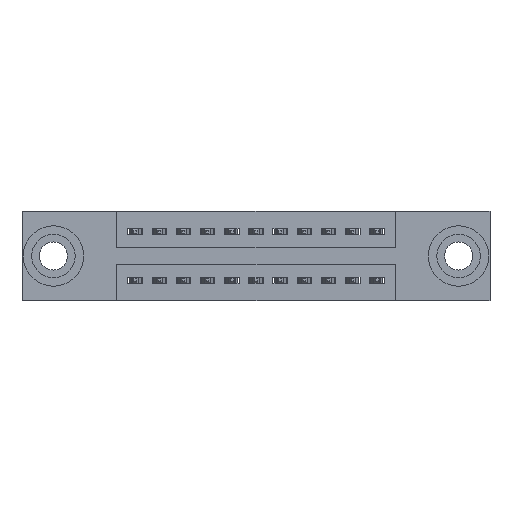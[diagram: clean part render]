
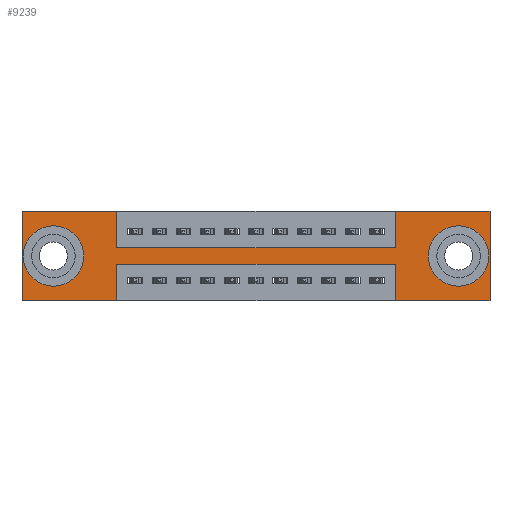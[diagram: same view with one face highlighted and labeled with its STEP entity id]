
A CAD part, front view. The second image highlights one B-rep face of the part: STEP entity #9239.
In plain terms, the highlighted planar face has unit normal (0, -1, 0).
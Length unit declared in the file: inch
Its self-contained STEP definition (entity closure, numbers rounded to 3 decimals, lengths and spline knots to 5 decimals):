
#27 = ORIENTED_EDGE ( 'NONE', *, *, #8693, .F. ) ;
#55 = LINE ( 'NONE', #4113, #10919 ) ;
#176 = CARTESIAN_POINT ( 'NONE',  ( 1.805, 0., -0.263 ) ) ;
#254 = DIRECTION ( 'NONE',  ( 0., 1., 0. ) ) ;
#573 = EDGE_CURVE ( 'NONE', #13334, #4779, #3829, .T. ) ;
#796 = VERTEX_POINT ( 'NONE', #4320 ) ;
#838 = VECTOR ( 'NONE', #10390, 39.37008 ) ;
#892 = CARTESIAN_POINT ( 'NONE',  ( 0.3925, 0., -0.22 ) ) ;
#930 = CARTESIAN_POINT ( 'NONE',  ( 0., 0., 0. ) ) ;
#1156 = CARTESIAN_POINT ( 'NONE',  ( 0., 0., -0.37 ) ) ;
#1163 = EDGE_LOOP ( 'NONE', ( #5607, #6394 ) ) ;
#1349 = VERTEX_POINT ( 'NONE', #5941 ) ;
#1378 = DIRECTION ( 'NONE',  ( 0., 0., 1. ) ) ;
#1392 = EDGE_CURVE ( 'NONE', #10731, #13496, #9071, .T. ) ;
#1837 = CARTESIAN_POINT ( 'NONE',  ( 0.3925, 0., -0.15 ) ) ;
#1851 = DIRECTION ( 'NONE',  ( 1., 0., 0. ) ) ;
#1896 = EDGE_CURVE ( 'NONE', #3191, #8686, #5848, .T. ) ;
#1983 = ORIENTED_EDGE ( 'NONE', *, *, #9876, .F. ) ;
#2109 = CARTESIAN_POINT ( 'NONE',  ( 0.3925, 0., -0.15 ) ) ;
#2482 = EDGE_CURVE ( 'NONE', #2484, #11523, #7688, .T. ) ;
#2484 = VERTEX_POINT ( 'NONE', #2109 ) ;
#2642 = CIRCLE ( 'NONE', #4278, 0.078 ) ;
#2674 = ORIENTED_EDGE ( 'NONE', *, *, #5339, .F. ) ;
#2842 = ORIENTED_EDGE ( 'NONE', *, *, #573, .F. ) ;
#2882 = EDGE_CURVE ( 'NONE', #11814, #8752, #55, .T. ) ;
#3098 = VERTEX_POINT ( 'NONE', #6327 ) ;
#3191 = VERTEX_POINT ( 'NONE', #176 ) ;
#3292 = VECTOR ( 'NONE', #3511, 39.37008 ) ;
#3360 = EDGE_CURVE ( 'NONE', #13496, #4398, #11506, .T. ) ;
#3401 = DIRECTION ( 'NONE',  ( 0., 0., -1. ) ) ;
#3511 = DIRECTION ( 'NONE',  ( 1., 0., 0. ) ) ;
#3582 = FACE_OUTER_BOUND ( 'NONE', #8146, .T. ) ;
#3628 = CARTESIAN_POINT ( 'NONE',  ( 0.3925, 0., 0. ) ) ;
#3829 = LINE ( 'NONE', #10468, #838 ) ;
#4071 = EDGE_CURVE ( 'NONE', #11523, #10731, #13058, .T. ) ;
#4113 = CARTESIAN_POINT ( 'NONE',  ( 0., 0., -0.37 ) ) ;
#4177 = CARTESIAN_POINT ( 'NONE',  ( 1.5425, 0., -0.15 ) ) ;
#4278 = AXIS2_PLACEMENT_3D ( 'NONE', #9083, #9059, #9030 ) ;
#4320 = CARTESIAN_POINT ( 'NONE',  ( 0.3925, 0., 0. ) ) ;
#4358 = CARTESIAN_POINT ( 'NONE',  ( 0., 0., -0.37 ) ) ;
#4398 = VERTEX_POINT ( 'NONE', #5504 ) ;
#4517 = DIRECTION ( 'NONE',  ( -1., 0., 0. ) ) ;
#4561 = LINE ( 'NONE', #8223, #6668 ) ;
#4618 = ORIENTED_EDGE ( 'NONE', *, *, #2482, .F. ) ;
#4779 = VERTEX_POINT ( 'NONE', #892 ) ;
#5067 = CARTESIAN_POINT ( 'NONE',  ( 0.3925, 0., -0.37 ) ) ;
#5075 = CARTESIAN_POINT ( 'NONE',  ( 1.5425, 0., 0. ) ) ;
#5090 = DIRECTION ( 'NONE',  ( 0., 0., -1. ) ) ;
#5096 = DIRECTION ( 'NONE',  ( 0., 1., 0. ) ) ;
#5107 = CARTESIAN_POINT ( 'NONE',  ( 1.805, 0., -0.185 ) ) ;
#5154 = AXIS2_PLACEMENT_3D ( 'NONE', #1156, #9513, #3401 ) ;
#5237 = EDGE_CURVE ( 'NONE', #3098, #6675, #2642, .T. ) ;
#5339 = EDGE_CURVE ( 'NONE', #4398, #6789, #4561, .T. ) ;
#5445 = ORIENTED_EDGE ( 'NONE', *, *, #7848, .F. ) ;
#5484 = CIRCLE ( 'NONE', #5872, 0.078 ) ;
#5504 = CARTESIAN_POINT ( 'NONE',  ( 1.935, 0., -0.37 ) ) ;
#5607 = ORIENTED_EDGE ( 'NONE', *, *, #9291, .T. ) ;
#5729 = DIRECTION ( 'NONE',  ( 0., 1., 0. ) ) ;
#5848 = CIRCLE ( 'NONE', #9488, 0.078 ) ;
#5872 = AXIS2_PLACEMENT_3D ( 'NONE', #11615, #5729, #12656 ) ;
#5941 = CARTESIAN_POINT ( 'NONE',  ( 0., 0., 0. ) ) ;
#5956 = ORIENTED_EDGE ( 'NONE', *, *, #3360, .F. ) ;
#6174 = VECTOR ( 'NONE', #9669, 39.37008 ) ;
#6288 = VECTOR ( 'NONE', #12557, 39.37008 ) ;
#6327 = CARTESIAN_POINT ( 'NONE',  ( 0.13, 0., -0.263 ) ) ;
#6394 = ORIENTED_EDGE ( 'NONE', *, *, #1896, .T. ) ;
#6548 = DIRECTION ( 'NONE',  ( 0., 0., 1. ) ) ;
#6635 = CARTESIAN_POINT ( 'NONE',  ( 1.5425, 0., 0. ) ) ;
#6668 = VECTOR ( 'NONE', #8156, 39.37008 ) ;
#6675 = VERTEX_POINT ( 'NONE', #11117 ) ;
#6789 = VERTEX_POINT ( 'NONE', #12276 ) ;
#6810 = CARTESIAN_POINT ( 'NONE',  ( 0.13, 0., -0.185 ) ) ;
#6893 = CARTESIAN_POINT ( 'NONE',  ( 1.935, 0., 0. ) ) ;
#7376 = VECTOR ( 'NONE', #1851, 39.37008 ) ;
#7512 = VECTOR ( 'NONE', #7808, 39.37008 ) ;
#7574 = PLANE ( 'NONE',  #5154 ) ;
#7671 = VECTOR ( 'NONE', #11319, 39.37008 ) ;
#7688 = LINE ( 'NONE', #1837, #7376 ) ;
#7802 = DIRECTION ( 'NONE',  ( 0., 0., 1. ) ) ;
#7808 = DIRECTION ( 'NONE',  ( 0., 0., -1. ) ) ;
#7848 = EDGE_CURVE ( 'NONE', #4779, #11814, #12982, .T. ) ;
#8091 = ORIENTED_EDGE ( 'NONE', *, *, #1392, .F. ) ;
#8146 = EDGE_LOOP ( 'NONE', ( #5445, #2842, #1983, #2674, #5956, #8091, #11315, #4618, #10391, #13231, #27, #8570 ) ) ;
#8156 = DIRECTION ( 'NONE',  ( -1., 0., 0. ) ) ;
#8223 = CARTESIAN_POINT ( 'NONE',  ( 0., 0., -0.37 ) ) ;
#8570 = ORIENTED_EDGE ( 'NONE', *, *, #2882, .F. ) ;
#8605 = EDGE_LOOP ( 'NONE', ( #12283, #8711 ) ) ;
#8686 = VERTEX_POINT ( 'NONE', #13294 ) ;
#8693 = EDGE_CURVE ( 'NONE', #8752, #1349, #10257, .T. ) ;
#8711 = ORIENTED_EDGE ( 'NONE', *, *, #5237, .T. ) ;
#8751 = CARTESIAN_POINT ( 'NONE',  ( 1.5425, 0., -0.37 ) ) ;
#8752 = VERTEX_POINT ( 'NONE', #4358 ) ;
#8858 = VECTOR ( 'NONE', #1378, 39.37008 ) ;
#8938 = EDGE_CURVE ( 'NONE', #796, #2484, #12803, .T. ) ;
#9030 = DIRECTION ( 'NONE',  ( 0., 0., 1. ) ) ;
#9032 = FACE_BOUND ( 'NONE', #1163, .T. ) ;
#9059 = DIRECTION ( 'NONE',  ( 0., 1., 0. ) ) ;
#9071 = LINE ( 'NONE', #11192, #6174 ) ;
#9083 = CARTESIAN_POINT ( 'NONE',  ( 0.13, 0., -0.185 ) ) ;
#9239 = ADVANCED_FACE ( 'NONE', ( #9032, #11333, #3582 ), #7574, .T. ) ;
#9291 = EDGE_CURVE ( 'NONE', #8686, #3191, #5484, .T. ) ;
#9488 = AXIS2_PLACEMENT_3D ( 'NONE', #5107, #5096, #5090 ) ;
#9513 = DIRECTION ( 'NONE',  ( 0., -1., 0. ) ) ;
#9618 = CARTESIAN_POINT ( 'NONE',  ( 0.3925, 0., -0.37 ) ) ;
#9669 = DIRECTION ( 'NONE',  ( 1., 0., 0. ) ) ;
#9876 = EDGE_CURVE ( 'NONE', #6789, #13334, #13212, .T. ) ;
#10116 = AXIS2_PLACEMENT_3D ( 'NONE', #6810, #254, #7802 ) ;
#10257 = LINE ( 'NONE', #930, #7671 ) ;
#10364 = VECTOR ( 'NONE', #6548, 39.37008 ) ;
#10390 = DIRECTION ( 'NONE',  ( -1., 0., 0. ) ) ;
#10391 = ORIENTED_EDGE ( 'NONE', *, *, #8938, .F. ) ;
#10468 = CARTESIAN_POINT ( 'NONE',  ( 0.3925, 0., -0.22 ) ) ;
#10545 = EDGE_CURVE ( 'NONE', #6675, #3098, #11318, .T. ) ;
#10585 = CARTESIAN_POINT ( 'NONE',  ( 0., 0., 0. ) ) ;
#10616 = VECTOR ( 'NONE', #12023, 39.37008 ) ;
#10731 = VERTEX_POINT ( 'NONE', #5075 ) ;
#10919 = VECTOR ( 'NONE', #4517, 39.37008 ) ;
#11117 = CARTESIAN_POINT ( 'NONE',  ( 0.13, 0., -0.107 ) ) ;
#11192 = CARTESIAN_POINT ( 'NONE',  ( 0., 0., 0. ) ) ;
#11315 = ORIENTED_EDGE ( 'NONE', *, *, #4071, .F. ) ;
#11318 = CIRCLE ( 'NONE', #10116, 0.078 ) ;
#11319 = DIRECTION ( 'NONE',  ( 0., 0., 1. ) ) ;
#11333 = FACE_BOUND ( 'NONE', #8605, .T. ) ;
#11506 = LINE ( 'NONE', #12587, #6288 ) ;
#11523 = VERTEX_POINT ( 'NONE', #4177 ) ;
#11615 = CARTESIAN_POINT ( 'NONE',  ( 1.805, 0., -0.185 ) ) ;
#11724 = LINE ( 'NONE', #10585, #3292 ) ;
#11814 = VERTEX_POINT ( 'NONE', #9618 ) ;
#12023 = DIRECTION ( 'NONE',  ( 0., 0., -1. ) ) ;
#12276 = CARTESIAN_POINT ( 'NONE',  ( 1.5425, 0., -0.37 ) ) ;
#12283 = ORIENTED_EDGE ( 'NONE', *, *, #10545, .T. ) ;
#12487 = CARTESIAN_POINT ( 'NONE',  ( 1.5425, 0., -0.22 ) ) ;
#12557 = DIRECTION ( 'NONE',  ( 0., 0., -1. ) ) ;
#12587 = CARTESIAN_POINT ( 'NONE',  ( 1.935, 0., 0. ) ) ;
#12656 = DIRECTION ( 'NONE',  ( 0., 0., -1. ) ) ;
#12803 = LINE ( 'NONE', #3628, #7512 ) ;
#12982 = LINE ( 'NONE', #5067, #10616 ) ;
#13058 = LINE ( 'NONE', #6635, #10364 ) ;
#13212 = LINE ( 'NONE', #8751, #8858 ) ;
#13231 = ORIENTED_EDGE ( 'NONE', *, *, #13368, .F. ) ;
#13294 = CARTESIAN_POINT ( 'NONE',  ( 1.805, 0., -0.107 ) ) ;
#13334 = VERTEX_POINT ( 'NONE', #12487 ) ;
#13368 = EDGE_CURVE ( 'NONE', #1349, #796, #11724, .T. ) ;
#13496 = VERTEX_POINT ( 'NONE', #6893 ) ;
